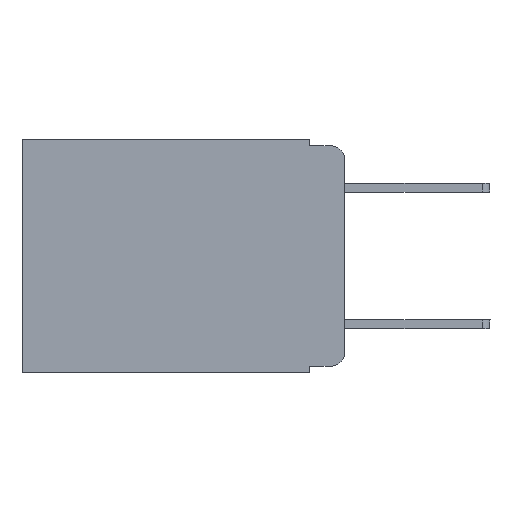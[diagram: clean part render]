
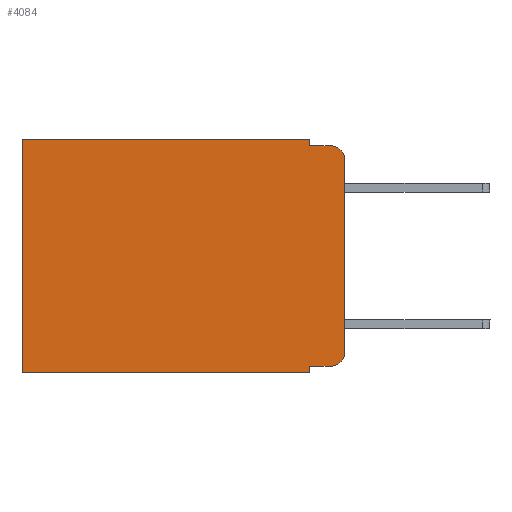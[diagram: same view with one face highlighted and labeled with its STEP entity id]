
A CAD part, left-side view. The second image highlights one B-rep face of the part: STEP entity #4084.
In plain terms, the highlighted planar face has unit normal (-1, 0, 0).
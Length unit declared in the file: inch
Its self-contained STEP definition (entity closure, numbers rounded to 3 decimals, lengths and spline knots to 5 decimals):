
#258 = EDGE_CURVE ( 'NONE', #13352, #2882, #1742, .T. ) ;
#357 = ORIENTED_EDGE ( 'NONE', *, *, #258, .T. ) ;
#409 = DIRECTION ( 'NONE',  ( 0., -1., 0. ) ) ;
#720 = CARTESIAN_POINT ( 'NONE',  ( 0.298, 0., 0. ) ) ;
#805 = LINE ( 'NONE', #4392, #9677 ) ;
#1021 = CARTESIAN_POINT ( 'NONE',  ( 0.298, 0.051, -0.01 ) ) ;
#1484 = DIRECTION ( 'NONE',  ( 0., 0., -1. ) ) ;
#1576 = LINE ( 'NONE', #12394, #7033 ) ;
#1598 = CARTESIAN_POINT ( 'NONE',  ( 0.298, 0.02, -0.333 ) ) ;
#1742 = CIRCLE ( 'NONE', #13031, 0.02 ) ;
#1802 = DIRECTION ( 'NONE',  ( 0., -1., 0. ) ) ;
#1817 = CARTESIAN_POINT ( 'NONE',  ( 0.298, 0., 0. ) ) ;
#1826 = DIRECTION ( 'NONE',  ( 1., 0., 0. ) ) ;
#1860 = CARTESIAN_POINT ( 'NONE',  ( 0.298, 0.02, -0.01 ) ) ;
#1874 = ORIENTED_EDGE ( 'NONE', *, *, #2216, .F. ) ;
#2045 = CARTESIAN_POINT ( 'NONE',  ( 0.298, 0.051, 0. ) ) ;
#2102 = EDGE_CURVE ( 'NONE', #10829, #7380, #13066, .T. ) ;
#2158 = VERTEX_POINT ( 'NONE', #2045 ) ;
#2204 = CARTESIAN_POINT ( 'NONE',  ( 0.298, 0.051, -0.01 ) ) ;
#2216 = EDGE_CURVE ( 'NONE', #11686, #8034, #2528, .T. ) ;
#2528 = LINE ( 'NONE', #11045, #7992 ) ;
#2703 = CIRCLE ( 'NONE', #6267, 0.02 ) ;
#2857 = CARTESIAN_POINT ( 'NONE',  ( 0.298, 0.051, -0.333 ) ) ;
#2882 = VERTEX_POINT ( 'NONE', #10916 ) ;
#2931 = ORIENTED_EDGE ( 'NONE', *, *, #5291, .T. ) ;
#3061 = CARTESIAN_POINT ( 'NONE',  ( 0.298, 0.473, 0. ) ) ;
#3161 = EDGE_CURVE ( 'NONE', #7552, #13352, #12699, .T. ) ;
#3589 = LINE ( 'NONE', #3061, #9213 ) ;
#4084 = ADVANCED_FACE ( 'NONE', ( #12346 ), #9171, .F. ) ;
#4392 = CARTESIAN_POINT ( 'NONE',  ( 0.298, 0.051, 0. ) ) ;
#4609 = CARTESIAN_POINT ( 'NONE',  ( 0.298, 0.051, -0.343 ) ) ;
#5071 = VERTEX_POINT ( 'NONE', #10969 ) ;
#5102 = DIRECTION ( 'NONE',  ( 0., 0., -1. ) ) ;
#5129 = EDGE_CURVE ( 'NONE', #2158, #10829, #805, .T. ) ;
#5183 = CARTESIAN_POINT ( 'NONE',  ( 0.298, 0.473, 0. ) ) ;
#5291 = EDGE_CURVE ( 'NONE', #5071, #7380, #2703, .T. ) ;
#5491 = VECTOR ( 'NONE', #8870, 39.37008 ) ;
#5776 = ORIENTED_EDGE ( 'NONE', *, *, #2102, .F. ) ;
#5866 = DIRECTION ( 'NONE',  ( -1., 0., 0. ) ) ;
#5934 = VECTOR ( 'NONE', #7068, 39.37008 ) ;
#6267 = AXIS2_PLACEMENT_3D ( 'NONE', #12376, #5866, #1484 ) ;
#6376 = EDGE_LOOP ( 'NONE', ( #10284, #2931, #5776, #10043, #11074, #12481, #1874, #7212, #13726, #357 ) ) ;
#7033 = VECTOR ( 'NONE', #13561, 39.37008 ) ;
#7068 = DIRECTION ( 'NONE',  ( 0., 0., -1. ) ) ;
#7078 = AXIS2_PLACEMENT_3D ( 'NONE', #720, #1826, #12760 ) ;
#7212 = ORIENTED_EDGE ( 'NONE', *, *, #12540, .F. ) ;
#7223 = CARTESIAN_POINT ( 'NONE',  ( 0.298, 0.473, -0.343 ) ) ;
#7380 = VERTEX_POINT ( 'NONE', #1860 ) ;
#7552 = VERTEX_POINT ( 'NONE', #9673 ) ;
#7992 = VECTOR ( 'NONE', #13234, 39.37008 ) ;
#8034 = VERTEX_POINT ( 'NONE', #7223 ) ;
#8132 = VECTOR ( 'NONE', #1802, 39.37008 ) ;
#8400 = DIRECTION ( 'NONE',  ( 0., 0., -1. ) ) ;
#8870 = DIRECTION ( 'NONE',  ( 0., 1., 0. ) ) ;
#9171 = PLANE ( 'NONE',  #7078 ) ;
#9213 = VECTOR ( 'NONE', #8400, 39.37008 ) ;
#9271 = VERTEX_POINT ( 'NONE', #5183 ) ;
#9673 = CARTESIAN_POINT ( 'NONE',  ( 0.298, 0.051, -0.333 ) ) ;
#9677 = VECTOR ( 'NONE', #9890, 39.37008 ) ;
#9890 = DIRECTION ( 'NONE',  ( 0., 0., -1. ) ) ;
#10043 = ORIENTED_EDGE ( 'NONE', *, *, #5129, .F. ) ;
#10284 = ORIENTED_EDGE ( 'NONE', *, *, #11209, .F. ) ;
#10536 = CARTESIAN_POINT ( 'NONE',  ( 0.298, 0.02, -0.313 ) ) ;
#10829 = VERTEX_POINT ( 'NONE', #1021 ) ;
#10916 = CARTESIAN_POINT ( 'NONE',  ( 0.298, 0., -0.313 ) ) ;
#10969 = CARTESIAN_POINT ( 'NONE',  ( 0.298, 0., -0.03 ) ) ;
#11045 = CARTESIAN_POINT ( 'NONE',  ( 0.298, 0., -0.343 ) ) ;
#11074 = ORIENTED_EDGE ( 'NONE', *, *, #13831, .T. ) ;
#11209 = EDGE_CURVE ( 'NONE', #5071, #2882, #11386, .T. ) ;
#11385 = EDGE_CURVE ( 'NONE', #9271, #8034, #3589, .T. ) ;
#11386 = LINE ( 'NONE', #1817, #5934 ) ;
#11626 = DIRECTION ( 'NONE',  ( -1., 0., 0. ) ) ;
#11686 = VERTEX_POINT ( 'NONE', #4609 ) ;
#11951 = LINE ( 'NONE', #12011, #5491 ) ;
#12011 = CARTESIAN_POINT ( 'NONE',  ( 0.298, 0., 0. ) ) ;
#12346 = FACE_OUTER_BOUND ( 'NONE', #6376, .T. ) ;
#12376 = CARTESIAN_POINT ( 'NONE',  ( 0.298, 0.02, -0.03 ) ) ;
#12394 = CARTESIAN_POINT ( 'NONE',  ( 0.298, 0.051, 0. ) ) ;
#12481 = ORIENTED_EDGE ( 'NONE', *, *, #11385, .T. ) ;
#12540 = EDGE_CURVE ( 'NONE', #7552, #11686, #1576, .T. ) ;
#12699 = LINE ( 'NONE', #2857, #8132 ) ;
#12760 = DIRECTION ( 'NONE',  ( 0., 0., -1. ) ) ;
#12913 = VECTOR ( 'NONE', #409, 39.37008 ) ;
#13031 = AXIS2_PLACEMENT_3D ( 'NONE', #10536, #11626, #5102 ) ;
#13066 = LINE ( 'NONE', #2204, #12913 ) ;
#13234 = DIRECTION ( 'NONE',  ( 0., 1., 0. ) ) ;
#13352 = VERTEX_POINT ( 'NONE', #1598 ) ;
#13561 = DIRECTION ( 'NONE',  ( 0., 0., -1. ) ) ;
#13726 = ORIENTED_EDGE ( 'NONE', *, *, #3161, .T. ) ;
#13831 = EDGE_CURVE ( 'NONE', #2158, #9271, #11951, .T. ) ;
